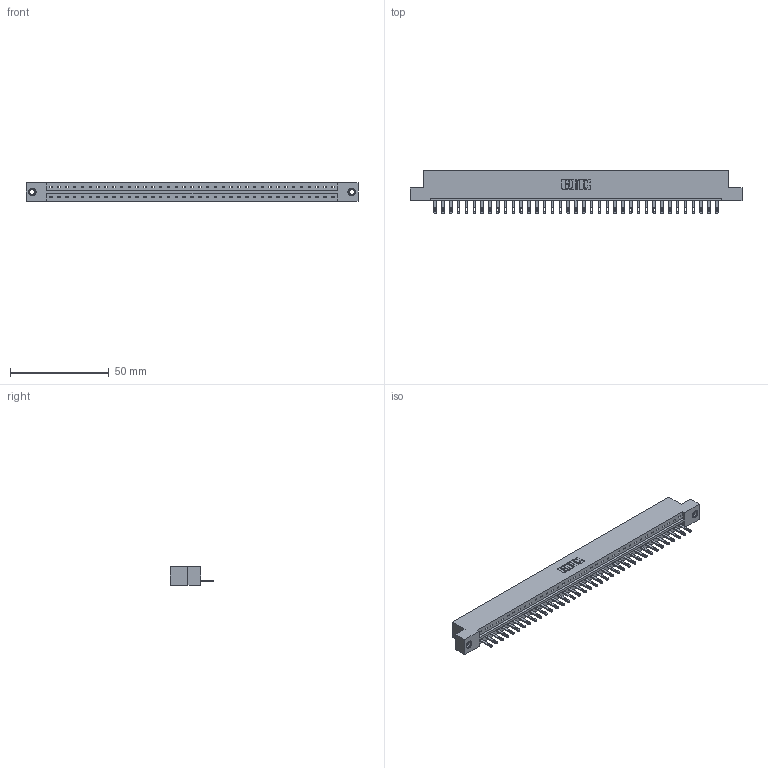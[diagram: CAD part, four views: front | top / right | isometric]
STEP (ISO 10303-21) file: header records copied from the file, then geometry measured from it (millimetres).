
FILE_DESCRIPTION (( 'STEP AP203' ), '1' );
FILE_NAME ('833-037-500-107.STEP', '2020-06-03T04:33:05', ( '' ), ( '' ), 'SwSTEP 2.0', 'SolidWorks 2020', '' );
FILE_SCHEMA (( 'CONFIG_CONTROL_DESIGN' ));
Length unit declared in the file: inch
Products named in the file (4): 345-292-001_345-293-100; 833 Part_Flush - .156 Dia - TI; 833-037-500-107; 345-250-001_345-250-005-103
Assembly tree (40 placements, depth 2):
  833-037-500-107
    833 Part_Flush - .156 Dia - TI
    345-292-001_345-293-100  x37
    345-250-001_345-250-005-103  x2
Bounding box: 168.15 x 21.85 x 9.4 mm (x, y, z)
Volume: 16886.8 mm3; surface area: 18365.9 mm2
Topology: 40 solids, 40 shells, 2172 faces, 6663 edges, 4434 vertices
Faces by surface type: plane 1434, cylinder 722, cone 12, torus 4
Entity records: 24382 total; most frequent: CARTESIAN_POINT 4188, ORIENTED_EDGE 4154, DIRECTION 3577, EDGE_CURVE 2077, LINE 1925, VECTOR 1925, VERTEX_POINT 1380, AXIS2_PLACEMENT_3D 826
